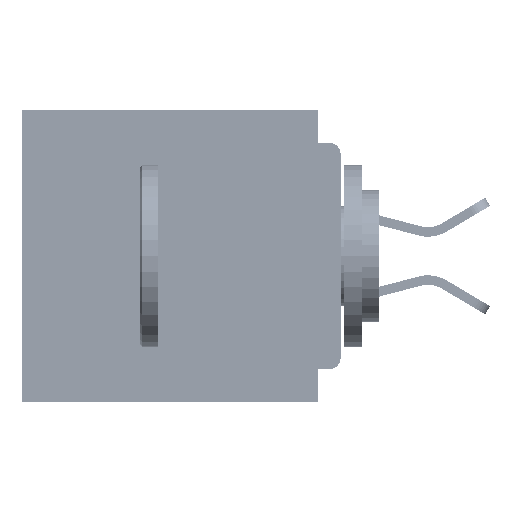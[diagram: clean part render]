
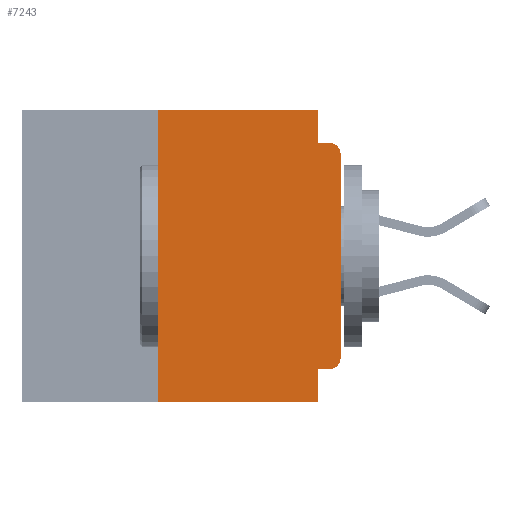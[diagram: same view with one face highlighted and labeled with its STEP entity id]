
A CAD part, left-side view. The second image highlights one B-rep face of the part: STEP entity #7243.
In plain terms, the highlighted planar face has unit normal (-1, 0, 0).
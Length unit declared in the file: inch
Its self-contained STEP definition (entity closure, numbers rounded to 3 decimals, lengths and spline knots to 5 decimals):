
#303 = ORIENTED_EDGE ( 'NONE', *, *, #37137, .F. ) ;
#387 = VECTOR ( 'NONE', #51838, 39.37008 ) ;
#1426 = FACE_OUTER_BOUND ( 'NONE', #1755, .T. ) ;
#1755 = EDGE_LOOP ( 'NONE', ( #60402, #18219, #7451, #303, #20490, #45571, #55457, #19312, #18519, #38691 ) ) ;
#1991 = DIRECTION ( 'NONE',  ( 0., 1., 0. ) ) ;
#2529 = CARTESIAN_POINT ( 'NONE',  ( 0., 0.25, -0.4 ) ) ;
#2868 = DIRECTION ( 'NONE',  ( 0., -1., 0. ) ) ;
#3307 = CARTESIAN_POINT ( 'NONE',  ( 0., 0.015, -0.06 ) ) ;
#5632 = DIRECTION ( 'NONE',  ( 0., -1., 0. ) ) ;
#6020 = CARTESIAN_POINT ( 'NONE',  ( 0., 0.031, 0. ) ) ;
#6373 = CARTESIAN_POINT ( 'NONE',  ( 0., 0., 0. ) ) ;
#7243 = ADVANCED_FACE ( 'NONE', ( #1426 ), #45110, .F. ) ;
#7451 = ORIENTED_EDGE ( 'NONE', *, *, #9928, .F. ) ;
#8387 = DIRECTION ( 'NONE',  ( 0., 0., -1. ) ) ;
#9928 = EDGE_CURVE ( 'NONE', #35724, #49486, #24979, .T. ) ;
#10822 = LINE ( 'NONE', #6373, #47291 ) ;
#11104 = CIRCLE ( 'NONE', #55499, 0.015 ) ;
#14640 = CARTESIAN_POINT ( 'NONE',  ( 0., 0., -0.34 ) ) ;
#15440 = DIRECTION ( 'NONE',  ( 1., 0., 0. ) ) ;
#15510 = CARTESIAN_POINT ( 'NONE',  ( 0., 0., -0.045 ) ) ;
#15590 = LINE ( 'NONE', #6020, #55000 ) ;
#16224 = VECTOR ( 'NONE', #48582, 39.37008 ) ;
#17128 = CARTESIAN_POINT ( 'NONE',  ( 0., 0.015, -0.34 ) ) ;
#18219 = ORIENTED_EDGE ( 'NONE', *, *, #24987, .T. ) ;
#18519 = ORIENTED_EDGE ( 'NONE', *, *, #28383, .F. ) ;
#19312 = ORIENTED_EDGE ( 'NONE', *, *, #24471, .F. ) ;
#20490 = ORIENTED_EDGE ( 'NONE', *, *, #34031, .F. ) ;
#20875 = VERTEX_POINT ( 'NONE', #54909 ) ;
#22173 = DIRECTION ( 'NONE',  ( 0., 0., -1. ) ) ;
#22439 = CARTESIAN_POINT ( 'NONE',  ( 0., 0.437, 0. ) ) ;
#23672 = CARTESIAN_POINT ( 'NONE',  ( 0., 0.031, -0.4 ) ) ;
#24276 = CARTESIAN_POINT ( 'NONE',  ( 0., 0.015, -0.045 ) ) ;
#24471 = EDGE_CURVE ( 'NONE', #20875, #56287, #57189, .T. ) ;
#24979 = LINE ( 'NONE', #15510, #34980 ) ;
#24987 = EDGE_CURVE ( 'NONE', #54075, #49486, #64032, .T. ) ;
#27250 = CARTESIAN_POINT ( 'NONE',  ( 0., 0.25, -0.4 ) ) ;
#28383 = EDGE_CURVE ( 'NONE', #45259, #20875, #58885, .T. ) ;
#32661 = VECTOR ( 'NONE', #1991, 39.37008 ) ;
#32718 = CARTESIAN_POINT ( 'NONE',  ( 0., 0.437, -0.4 ) ) ;
#34031 = EDGE_CURVE ( 'NONE', #39280, #61350, #53023, .T. ) ;
#34980 = VECTOR ( 'NONE', #5632, 39.37008 ) ;
#35724 = VERTEX_POINT ( 'NONE', #39640 ) ;
#35785 = DIRECTION ( 'NONE',  ( 0., 0., -1. ) ) ;
#37069 = DIRECTION ( 'NONE',  ( 0., -1., 0. ) ) ;
#37137 = EDGE_CURVE ( 'NONE', #61350, #35724, #15590, .T. ) ;
#38111 = DIRECTION ( 'NONE',  ( -1., 0., 0. ) ) ;
#38691 = ORIENTED_EDGE ( 'NONE', *, *, #43954, .T. ) ;
#39280 = VERTEX_POINT ( 'NONE', #61567 ) ;
#39467 = AXIS2_PLACEMENT_3D ( 'NONE', #3307, #38111, #8387 ) ;
#39640 = CARTESIAN_POINT ( 'NONE',  ( 0., 0.031, -0.045 ) ) ;
#40165 = AXIS2_PLACEMENT_3D ( 'NONE', #54743, #15440, #50066 ) ;
#41453 = VECTOR ( 'NONE', #37069, 39.37008 ) ;
#42140 = VECTOR ( 'NONE', #2868, 39.37008 ) ;
#43954 = EDGE_CURVE ( 'NONE', #45259, #63499, #11104, .T. ) ;
#45110 = PLANE ( 'NONE',  #40165 ) ;
#45259 = VERTEX_POINT ( 'NONE', #54729 ) ;
#45571 = ORIENTED_EDGE ( 'NONE', *, *, #53458, .F. ) ;
#46091 = DIRECTION ( 'NONE',  ( 0., 0., 1. ) ) ;
#47291 = VECTOR ( 'NONE', #46091, 39.37008 ) ;
#48582 = DIRECTION ( 'NONE',  ( 0., 0., -1. ) ) ;
#49486 = VERTEX_POINT ( 'NONE', #24276 ) ;
#49878 = VERTEX_POINT ( 'NONE', #2529 ) ;
#50066 = DIRECTION ( 'NONE',  ( 0., 0., -1. ) ) ;
#51505 = CARTESIAN_POINT ( 'NONE',  ( 0., 0., -0.355 ) ) ;
#51737 = DIRECTION ( 'NONE',  ( -1., 0., 0. ) ) ;
#51762 = CARTESIAN_POINT ( 'NONE',  ( 0., 0., -0.06 ) ) ;
#51838 = DIRECTION ( 'NONE',  ( 0., 0., 1. ) ) ;
#53023 = LINE ( 'NONE', #22439, #41453 ) ;
#53197 = LINE ( 'NONE', #27250, #387 ) ;
#53458 = EDGE_CURVE ( 'NONE', #49878, #39280, #53197, .T. ) ;
#54075 = VERTEX_POINT ( 'NONE', #51762 ) ;
#54729 = CARTESIAN_POINT ( 'NONE',  ( 0., 0.015, -0.355 ) ) ;
#54743 = CARTESIAN_POINT ( 'NONE',  ( 0., 0.437, 0. ) ) ;
#54909 = CARTESIAN_POINT ( 'NONE',  ( 0., 0.031, -0.355 ) ) ;
#55000 = VECTOR ( 'NONE', #35785, 39.37008 ) ;
#55228 = LINE ( 'NONE', #32718, #42140 ) ;
#55457 = ORIENTED_EDGE ( 'NONE', *, *, #62674, .T. ) ;
#55499 = AXIS2_PLACEMENT_3D ( 'NONE', #17128, #51737, #22173 ) ;
#56287 = VERTEX_POINT ( 'NONE', #23672 ) ;
#57189 = LINE ( 'NONE', #63375, #16224 ) ;
#58329 = EDGE_CURVE ( 'NONE', #63499, #54075, #10822, .T. ) ;
#58468 = CARTESIAN_POINT ( 'NONE',  ( 0., 0.031, 0. ) ) ;
#58885 = LINE ( 'NONE', #51505, #32661 ) ;
#60402 = ORIENTED_EDGE ( 'NONE', *, *, #58329, .T. ) ;
#61350 = VERTEX_POINT ( 'NONE', #58468 ) ;
#61567 = CARTESIAN_POINT ( 'NONE',  ( 0., 0.25, 0. ) ) ;
#62674 = EDGE_CURVE ( 'NONE', #49878, #56287, #55228, .T. ) ;
#63375 = CARTESIAN_POINT ( 'NONE',  ( 0., 0.031, -0.4 ) ) ;
#63499 = VERTEX_POINT ( 'NONE', #14640 ) ;
#64032 = CIRCLE ( 'NONE', #39467, 0.015 ) ;
